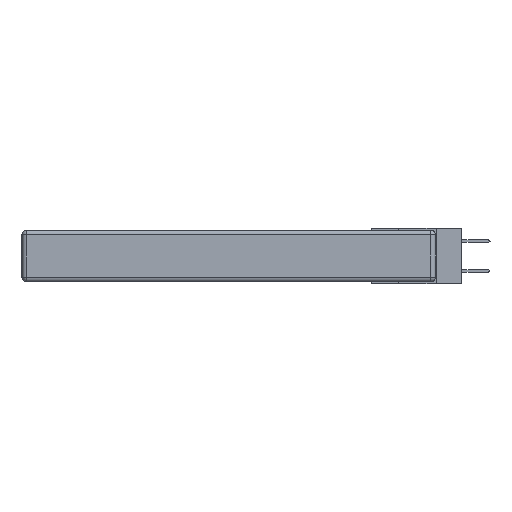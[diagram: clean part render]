
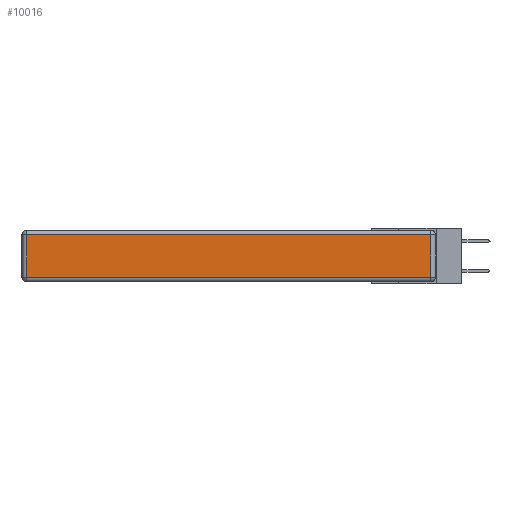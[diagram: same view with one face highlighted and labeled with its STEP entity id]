
A CAD part, left-side view. The second image highlights one B-rep face of the part: STEP entity #10016.
In plain terms, the highlighted planar face has unit normal (-1, 0, 0).
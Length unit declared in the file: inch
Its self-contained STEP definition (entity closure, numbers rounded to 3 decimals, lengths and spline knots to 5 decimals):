
#51 = VECTOR ( 'NONE', #4303, 39.37008 ) ;
#1142 = CARTESIAN_POINT ( 'NONE',  ( 0., 2.72, -0.313 ) ) ;
#1847 = DIRECTION ( 'NONE',  ( 0., 1., 0. ) ) ;
#2735 = FACE_OUTER_BOUND ( 'NONE', #13157, .T. ) ;
#2995 = ORIENTED_EDGE ( 'NONE', *, *, #10202, .T. ) ;
#3439 = EDGE_CURVE ( 'NONE', #9606, #5949, #8663, .T. ) ;
#3572 = CARTESIAN_POINT ( 'NONE',  ( 0., 2.75, -0.03 ) ) ;
#3893 = ORIENTED_EDGE ( 'NONE', *, *, #14131, .T. ) ;
#4203 = EDGE_CURVE ( 'NONE', #10826, #18313, #20994, .T. ) ;
#4303 = DIRECTION ( 'NONE',  ( 0., 0., 1. ) ) ;
#4716 = CARTESIAN_POINT ( 'NONE',  ( 0., 0., -0.343 ) ) ;
#5564 = CARTESIAN_POINT ( 'NONE',  ( 0., 0., -0.313 ) ) ;
#5949 = VERTEX_POINT ( 'NONE', #17697 ) ;
#7044 = DIRECTION ( 'NONE',  ( 0., -1., 0. ) ) ;
#7598 = ORIENTED_EDGE ( 'NONE', *, *, #4203, .T. ) ;
#7851 = CARTESIAN_POINT ( 'NONE',  ( 0., 0.03, -0.03 ) ) ;
#8663 = LINE ( 'NONE', #3572, #12520 ) ;
#9148 = CARTESIAN_POINT ( 'NONE',  ( 0., 0.03, -0.343 ) ) ;
#9606 = VERTEX_POINT ( 'NONE', #7851 ) ;
#10016 = ADVANCED_FACE ( 'NONE', ( #2735 ), #14416, .T. ) ;
#10202 = EDGE_CURVE ( 'NONE', #5949, #10826, #20394, .T. ) ;
#10427 = DIRECTION ( 'NONE',  ( 0., 0., -1. ) ) ;
#10793 = CARTESIAN_POINT ( 'NONE',  ( 0., 0.03, -0.313 ) ) ;
#10826 = VERTEX_POINT ( 'NONE', #1142 ) ;
#11501 = DIRECTION ( 'NONE',  ( 0., 0., 1. ) ) ;
#12510 = ORIENTED_EDGE ( 'NONE', *, *, #3439, .T. ) ;
#12520 = VECTOR ( 'NONE', #1847, 39.37008 ) ;
#13157 = EDGE_LOOP ( 'NONE', ( #7598, #3893, #12510, #2995 ) ) ;
#14131 = EDGE_CURVE ( 'NONE', #18313, #9606, #18645, .T. ) ;
#14207 = VECTOR ( 'NONE', #10427, 39.37008 ) ;
#14416 = PLANE ( 'NONE',  #16119 ) ;
#16119 = AXIS2_PLACEMENT_3D ( 'NONE', #4716, #18060, #11501 ) ;
#16840 = VECTOR ( 'NONE', #7044, 39.37008 ) ;
#17697 = CARTESIAN_POINT ( 'NONE',  ( 0., 2.72, -0.03 ) ) ;
#18060 = DIRECTION ( 'NONE',  ( -1., 0., 0. ) ) ;
#18313 = VERTEX_POINT ( 'NONE', #10793 ) ;
#18645 = LINE ( 'NONE', #9148, #51 ) ;
#19187 = CARTESIAN_POINT ( 'NONE',  ( 0., 2.72, -0.343 ) ) ;
#20394 = LINE ( 'NONE', #19187, #14207 ) ;
#20994 = LINE ( 'NONE', #5564, #16840 ) ;
